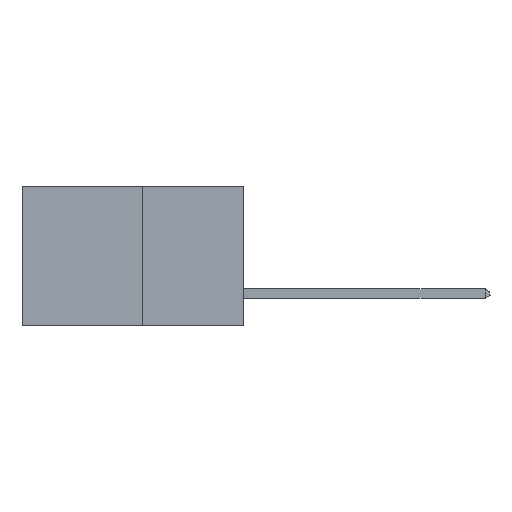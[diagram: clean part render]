
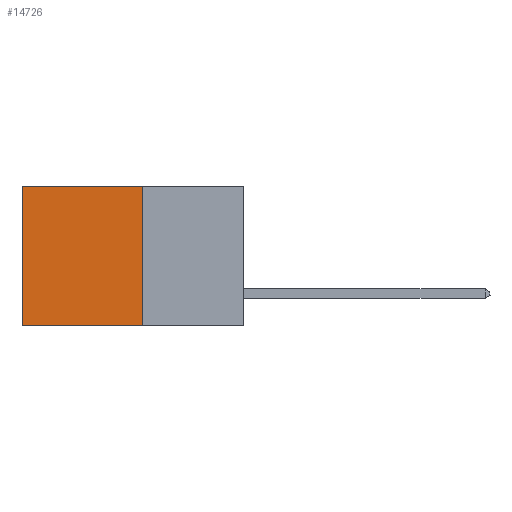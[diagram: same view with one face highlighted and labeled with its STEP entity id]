
A CAD part, left-side view. The second image highlights one B-rep face of the part: STEP entity #14726.
In plain terms, the highlighted planar face has unit normal (-1, 0, 0).
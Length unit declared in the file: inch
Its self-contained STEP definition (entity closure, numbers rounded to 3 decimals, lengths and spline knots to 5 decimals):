
#158 = DIRECTION ( 'NONE',  ( 1., 0., 0. ) ) ;
#169 = EDGE_CURVE ( 'NONE', #14190, #14435, #5044, .T. ) ;
#1419 = AXIS2_PLACEMENT_3D ( 'NONE', #7290, #158, #8458 ) ;
#1966 = EDGE_CURVE ( 'NONE', #14190, #9700, #5942, .T. ) ;
#3084 = CARTESIAN_POINT ( 'NONE',  ( 0.277, 0.59, 0. ) ) ;
#3115 = VERTEX_POINT ( 'NONE', #6061 ) ;
#3203 = CARTESIAN_POINT ( 'NONE',  ( 0.277, 0.27, 0. ) ) ;
#3536 = ORIENTED_EDGE ( 'NONE', *, *, #4218, .T. ) ;
#3691 = PLANE ( 'NONE',  #1419 ) ;
#4218 = EDGE_CURVE ( 'NONE', #14435, #3115, #8290, .T. ) ;
#5044 = LINE ( 'NONE', #3203, #10975 ) ;
#5080 = CARTESIAN_POINT ( 'NONE',  ( 0.277, 0.27, -0.37 ) ) ;
#5942 = LINE ( 'NONE', #5080, #12535 ) ;
#6061 = CARTESIAN_POINT ( 'NONE',  ( 0.277, 0.59, -0.37 ) ) ;
#6407 = DIRECTION ( 'NONE',  ( 0., 0., -1. ) ) ;
#7290 = CARTESIAN_POINT ( 'NONE',  ( 0.277, 0.27, -0.37 ) ) ;
#7556 = ORIENTED_EDGE ( 'NONE', *, *, #1966, .F. ) ;
#8290 = LINE ( 'NONE', #14347, #14784 ) ;
#8458 = DIRECTION ( 'NONE',  ( 0., 0., -1. ) ) ;
#9700 = VERTEX_POINT ( 'NONE', #10654 ) ;
#10313 = DIRECTION ( 'NONE',  ( 0., 1., 0. ) ) ;
#10441 = VECTOR ( 'NONE', #12286, 39.37008 ) ;
#10494 = ORIENTED_EDGE ( 'NONE', *, *, #11592, .F. ) ;
#10654 = CARTESIAN_POINT ( 'NONE',  ( 0.277, 0.27, -0.37 ) ) ;
#10834 = LINE ( 'NONE', #11156, #10441 ) ;
#10975 = VECTOR ( 'NONE', #10313, 39.37008 ) ;
#11156 = CARTESIAN_POINT ( 'NONE',  ( 0.277, 0.27, -0.37 ) ) ;
#11592 = EDGE_CURVE ( 'NONE', #9700, #3115, #10834, .T. ) ;
#12238 = ORIENTED_EDGE ( 'NONE', *, *, #169, .T. ) ;
#12286 = DIRECTION ( 'NONE',  ( 0., 1., 0. ) ) ;
#12535 = VECTOR ( 'NONE', #6407, 39.37008 ) ;
#12746 = CARTESIAN_POINT ( 'NONE',  ( 0.277, 0.27, 0. ) ) ;
#13848 = EDGE_LOOP ( 'NONE', ( #3536, #10494, #7556, #12238 ) ) ;
#14190 = VERTEX_POINT ( 'NONE', #12746 ) ;
#14269 = FACE_OUTER_BOUND ( 'NONE', #13848, .T. ) ;
#14318 = DIRECTION ( 'NONE',  ( 0., 0., -1. ) ) ;
#14347 = CARTESIAN_POINT ( 'NONE',  ( 0.277, 0.59, -0.37 ) ) ;
#14435 = VERTEX_POINT ( 'NONE', #3084 ) ;
#14726 = ADVANCED_FACE ( 'NONE', ( #14269 ), #3691, .F. ) ;
#14784 = VECTOR ( 'NONE', #14318, 39.37008 ) ;
